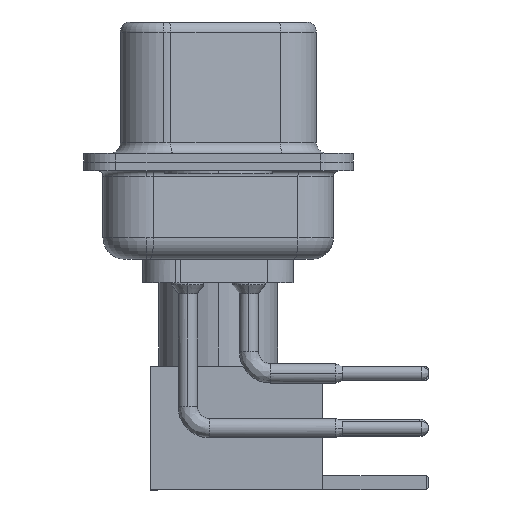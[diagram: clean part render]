
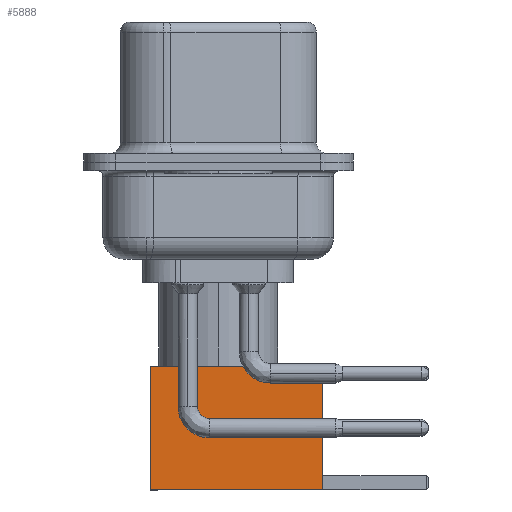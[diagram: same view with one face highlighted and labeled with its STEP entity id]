
A CAD part, left-side view. The second image highlights one B-rep face of the part: STEP entity #5888.
In plain terms, the highlighted face is planar.
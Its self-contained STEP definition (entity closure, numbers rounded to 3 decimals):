
#738 = ORIENTED_EDGE ( 'NONE', *, *, #1959, .T. ) ;
#1959 = EDGE_CURVE ( 'NONE', #11174, #13884, #18750, .T. ) ;
#4319 = VECTOR ( 'NONE', #14650, 1000. ) ;
#5453 = DIRECTION ( 'NONE',  ( 0., 0., -1. ) ) ;
#5888 = ADVANCED_FACE ( 'NONE', ( #26810 ), #27079, .T. ) ;
#7618 = DIRECTION ( 'NONE',  ( 0., 1., 0. ) ) ;
#8407 = CARTESIAN_POINT ( 'NONE',  ( 0., 2.875, 8. ) ) ;
#8479 = ORIENTED_EDGE ( 'NONE', *, *, #21815, .T. ) ;
#9368 = DIRECTION ( 'NONE',  ( 0., 0., 1. ) ) ;
#9999 = LINE ( 'NONE', #16272, #23494 ) ;
#10956 = DIRECTION ( 'NONE',  ( 0., 0., -1. ) ) ;
#11174 = VERTEX_POINT ( 'NONE', #27799 ) ;
#12613 = EDGE_CURVE ( 'NONE', #25881, #13884, #12810, .T. ) ;
#12810 = LINE ( 'NONE', #15376, #18013 ) ;
#13258 = CARTESIAN_POINT ( 'NONE',  ( -2.875, 2.875, 0. ) ) ;
#13884 = VERTEX_POINT ( 'NONE', #13258 ) ;
#14650 = DIRECTION ( 'NONE',  ( -1., 0., 0. ) ) ;
#15376 = CARTESIAN_POINT ( 'NONE',  ( -2.875, 2.875, 0. ) ) ;
#16272 = CARTESIAN_POINT ( 'NONE',  ( 2.875, 2.875, 0. ) ) ;
#16504 = AXIS2_PLACEMENT_3D ( 'NONE', #20417, #7618, #9368 ) ;
#16649 = EDGE_LOOP ( 'NONE', ( #8479, #738, #18595, #16826 ) ) ;
#16826 = ORIENTED_EDGE ( 'NONE', *, *, #25043, .F. ) ;
#17792 = VECTOR ( 'NONE', #21169, 1000. ) ;
#18013 = VECTOR ( 'NONE', #10956, 1000. ) ;
#18595 = ORIENTED_EDGE ( 'NONE', *, *, #12613, .F. ) ;
#18750 = LINE ( 'NONE', #23131, #4319 ) ;
#20417 = CARTESIAN_POINT ( 'NONE',  ( 2.875, 2.875, 0. ) ) ;
#21169 = DIRECTION ( 'NONE',  ( -1., 0., 0. ) ) ;
#21815 = EDGE_CURVE ( 'NONE', #25498, #11174, #9999, .T. ) ;
#23131 = CARTESIAN_POINT ( 'NONE',  ( 0., 2.875, 0. ) ) ;
#23494 = VECTOR ( 'NONE', #5453, 1000. ) ;
#23558 = CARTESIAN_POINT ( 'NONE',  ( 2.875, 2.875, 8. ) ) ;
#25043 = EDGE_CURVE ( 'NONE', #25498, #25881, #25590, .T. ) ;
#25498 = VERTEX_POINT ( 'NONE', #23558 ) ;
#25590 = LINE ( 'NONE', #8407, #17792 ) ;
#25719 = CARTESIAN_POINT ( 'NONE',  ( -2.875, 2.875, 8. ) ) ;
#25881 = VERTEX_POINT ( 'NONE', #25719 ) ;
#26810 = FACE_OUTER_BOUND ( 'NONE', #16649, .T. ) ;
#27079 = PLANE ( 'NONE',  #16504 ) ;
#27799 = CARTESIAN_POINT ( 'NONE',  ( 2.875, 2.875, 0. ) ) ;
